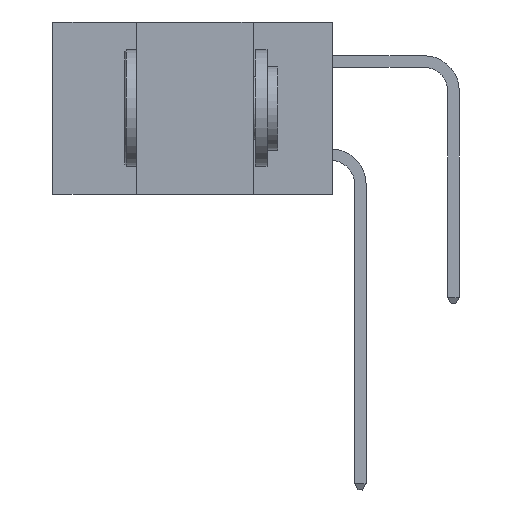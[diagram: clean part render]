
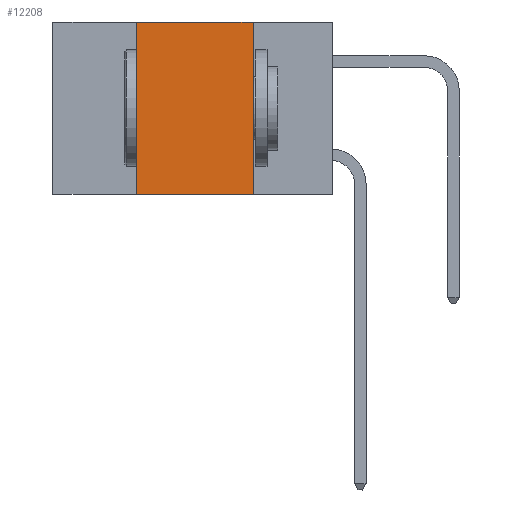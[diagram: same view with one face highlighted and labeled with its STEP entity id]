
A CAD part, left-side view. The second image highlights one B-rep face of the part: STEP entity #12208.
In plain terms, the highlighted planar face has unit normal (-1, 0, 0).
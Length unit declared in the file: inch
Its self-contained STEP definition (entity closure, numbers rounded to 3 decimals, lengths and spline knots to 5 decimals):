
#227 = CARTESIAN_POINT ( 'NONE',  ( 0., 0.42, -0.37 ) ) ;
#278 = CARTESIAN_POINT ( 'NONE',  ( 0., 0.42, 0. ) ) ;
#1457 = DIRECTION ( 'NONE',  ( 0., -1., 0. ) ) ;
#1614 = VECTOR ( 'NONE', #1457, 39.37008 ) ;
#2459 = CARTESIAN_POINT ( 'NONE',  ( 0., 0.17, 0. ) ) ;
#3822 = VERTEX_POINT ( 'NONE', #278 ) ;
#4185 = EDGE_CURVE ( 'NONE', #5623, #3822, #15674, .T. ) ;
#5191 = DIRECTION ( 'NONE',  ( 0., 0., 1. ) ) ;
#5623 = VERTEX_POINT ( 'NONE', #227 ) ;
#6083 = EDGE_CURVE ( 'NONE', #3822, #19250, #9354, .T. ) ;
#6954 = CARTESIAN_POINT ( 'NONE',  ( 0., 0.17, -0.37 ) ) ;
#7324 = EDGE_CURVE ( 'NONE', #5623, #21186, #18424, .T. ) ;
#7512 = EDGE_LOOP ( 'NONE', ( #15845, #17954, #19760, #23376 ) ) ;
#8185 = CARTESIAN_POINT ( 'NONE',  ( 0., 0.6, 0. ) ) ;
#9254 = AXIS2_PLACEMENT_3D ( 'NONE', #8185, #20909, #10708 ) ;
#9354 = LINE ( 'NONE', #16015, #16485 ) ;
#10708 = DIRECTION ( 'NONE',  ( 0., 0., -1. ) ) ;
#12208 = ADVANCED_FACE ( 'NONE', ( #18341 ), #22649, .F. ) ;
#14457 = VECTOR ( 'NONE', #15354, 39.37008 ) ;
#14936 = EDGE_CURVE ( 'NONE', #19250, #21186, #19324, .T. ) ;
#15354 = DIRECTION ( 'NONE',  ( 0., 0., -1. ) ) ;
#15674 = LINE ( 'NONE', #22863, #21938 ) ;
#15752 = CARTESIAN_POINT ( 'NONE',  ( 0., 0.6, -0.37 ) ) ;
#15845 = ORIENTED_EDGE ( 'NONE', *, *, #14936, .F. ) ;
#16015 = CARTESIAN_POINT ( 'NONE',  ( 0., 0.6, 0. ) ) ;
#16485 = VECTOR ( 'NONE', #23087, 39.37008 ) ;
#16881 = CARTESIAN_POINT ( 'NONE',  ( 0., 0.17, 0. ) ) ;
#17954 = ORIENTED_EDGE ( 'NONE', *, *, #6083, .F. ) ;
#18341 = FACE_OUTER_BOUND ( 'NONE', #7512, .T. ) ;
#18424 = LINE ( 'NONE', #15752, #1614 ) ;
#19250 = VERTEX_POINT ( 'NONE', #2459 ) ;
#19324 = LINE ( 'NONE', #16881, #14457 ) ;
#19760 = ORIENTED_EDGE ( 'NONE', *, *, #4185, .F. ) ;
#20909 = DIRECTION ( 'NONE',  ( 1., 0., 0. ) ) ;
#21186 = VERTEX_POINT ( 'NONE', #6954 ) ;
#21938 = VECTOR ( 'NONE', #5191, 39.37008 ) ;
#22649 = PLANE ( 'NONE',  #9254 ) ;
#22863 = CARTESIAN_POINT ( 'NONE',  ( 0., 0.42, 0. ) ) ;
#23087 = DIRECTION ( 'NONE',  ( 0., -1., 0. ) ) ;
#23376 = ORIENTED_EDGE ( 'NONE', *, *, #7324, .T. ) ;
